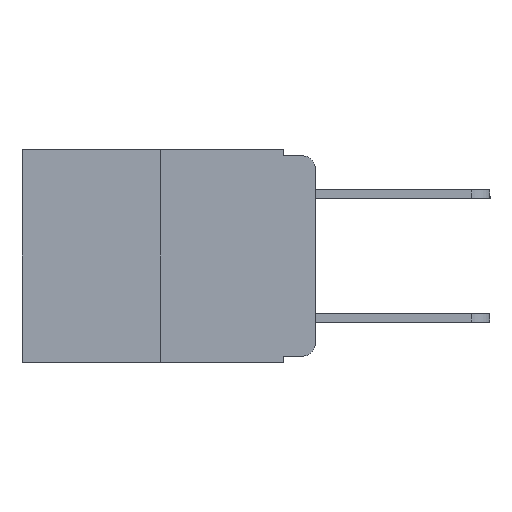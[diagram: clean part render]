
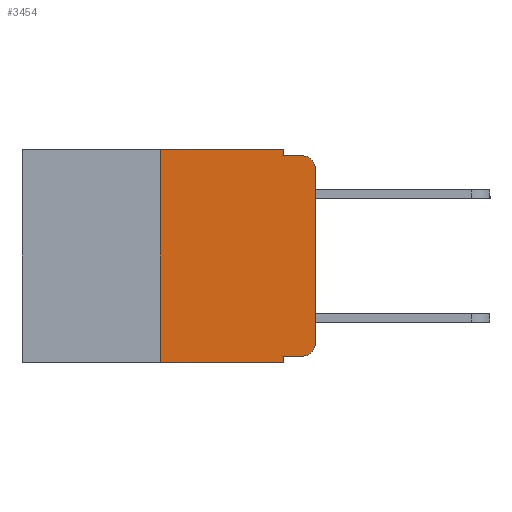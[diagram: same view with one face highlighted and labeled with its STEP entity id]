
A CAD part, left-side view. The second image highlights one B-rep face of the part: STEP entity #3454.
In plain terms, the highlighted planar face has unit normal (-1, 0, 0).
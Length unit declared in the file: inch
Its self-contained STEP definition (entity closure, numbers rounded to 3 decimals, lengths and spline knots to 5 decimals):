
#8 = CIRCLE ( 'NONE', #318, 0.02 ) ;
#318 = AXIS2_PLACEMENT_3D ( 'NONE', #6564, #405, #7449 ) ;
#341 = AXIS2_PLACEMENT_3D ( 'NONE', #9063, #3647, #9810 ) ;
#405 = DIRECTION ( 'NONE',  ( -1., 0., 0. ) ) ;
#509 = CARTESIAN_POINT ( 'NONE',  ( 0., 0.473, 0. ) ) ;
#791 = PLANE ( 'NONE',  #5399 ) ;
#895 = ORIENTED_EDGE ( 'NONE', *, *, #9069, .F. ) ;
#1317 = VERTEX_POINT ( 'NONE', #4248 ) ;
#1513 = VERTEX_POINT ( 'NONE', #5653 ) ;
#1748 = DIRECTION ( 'NONE',  ( 0., -1., 0. ) ) ;
#3040 = CARTESIAN_POINT ( 'NONE',  ( 0., 0.051, -0.343 ) ) ;
#3150 = LINE ( 'NONE', #4346, #7779 ) ;
#3346 = LINE ( 'NONE', #509, #10069 ) ;
#3454 = ADVANCED_FACE ( 'NONE', ( #8044 ), #791, .F. ) ;
#3488 = LINE ( 'NONE', #6900, #8137 ) ;
#3647 = DIRECTION ( 'NONE',  ( -1., 0., 0. ) ) ;
#3652 = LINE ( 'NONE', #7472, #8522 ) ;
#3686 = DIRECTION ( 'NONE',  ( 0., 0., -1. ) ) ;
#3776 = LINE ( 'NONE', #10562, #5989 ) ;
#3819 = EDGE_LOOP ( 'NONE', ( #5465, #4524, #5432, #895, #3895, #8691, #8847, #8886, #8919, #8930 ) ) ;
#3895 = ORIENTED_EDGE ( 'NONE', *, *, #9510, .F. ) ;
#4238 = VERTEX_POINT ( 'NONE', #5766 ) ;
#4248 = CARTESIAN_POINT ( 'NONE',  ( 0., 0.02, -0.01 ) ) ;
#4346 = CARTESIAN_POINT ( 'NONE',  ( 0., 0.473, -0.343 ) ) ;
#4377 = VERTEX_POINT ( 'NONE', #10115 ) ;
#4383 = VERTEX_POINT ( 'NONE', #6692 ) ;
#4524 = ORIENTED_EDGE ( 'NONE', *, *, #8584, .T. ) ;
#4530 = VERTEX_POINT ( 'NONE', #7323 ) ;
#4548 = LINE ( 'NONE', #5794, #7237 ) ;
#4826 = VECTOR ( 'NONE', #8921, 39.37008 ) ;
#5399 = AXIS2_PLACEMENT_3D ( 'NONE', #6695, #5581, #3686 ) ;
#5432 = ORIENTED_EDGE ( 'NONE', *, *, #8593, .F. ) ;
#5465 = ORIENTED_EDGE ( 'NONE', *, *, #9508, .T. ) ;
#5567 = LINE ( 'NONE', #10618, #7642 ) ;
#5581 = DIRECTION ( 'NONE',  ( 1., 0., 0. ) ) ;
#5653 = CARTESIAN_POINT ( 'NONE',  ( 0., 0.25, -0.343 ) ) ;
#5664 = DIRECTION ( 'NONE',  ( 0., 0., -1. ) ) ;
#5766 = CARTESIAN_POINT ( 'NONE',  ( 0., 0., -0.313 ) ) ;
#5794 = CARTESIAN_POINT ( 'NONE',  ( 0., 0.051, -0.333 ) ) ;
#5989 = VECTOR ( 'NONE', #11252, 39.37008 ) ;
#6550 = CIRCLE ( 'NONE', #341, 0.02 ) ;
#6564 = CARTESIAN_POINT ( 'NONE',  ( 0., 0.02, -0.313 ) ) ;
#6625 = DIRECTION ( 'NONE',  ( 0., 0., 1. ) ) ;
#6692 = CARTESIAN_POINT ( 'NONE',  ( 0., 0., -0.03 ) ) ;
#6695 = CARTESIAN_POINT ( 'NONE',  ( 0., 0.473, 0. ) ) ;
#6701 = CARTESIAN_POINT ( 'NONE',  ( 0., 0.25, 0. ) ) ;
#6900 = CARTESIAN_POINT ( 'NONE',  ( 0., 0.25, 0. ) ) ;
#7237 = VECTOR ( 'NONE', #11396, 39.37008 ) ;
#7323 = CARTESIAN_POINT ( 'NONE',  ( 0., 0.051, -0.333 ) ) ;
#7449 = DIRECTION ( 'NONE',  ( 0., 0., -1. ) ) ;
#7472 = CARTESIAN_POINT ( 'NONE',  ( 0., 0., 0. ) ) ;
#7642 = VECTOR ( 'NONE', #5664, 39.37008 ) ;
#7778 = DIRECTION ( 'NONE',  ( 0., 0., 1. ) ) ;
#7779 = VECTOR ( 'NONE', #11676, 39.37008 ) ;
#8044 = FACE_OUTER_BOUND ( 'NONE', #3819, .T. ) ;
#8137 = VECTOR ( 'NONE', #7778, 39.37008 ) ;
#8522 = VECTOR ( 'NONE', #6625, 39.37008 ) ;
#8584 = EDGE_CURVE ( 'NONE', #4383, #1317, #6550, .T. ) ;
#8593 = EDGE_CURVE ( 'NONE', #4377, #1317, #3776, .T. ) ;
#8608 = CARTESIAN_POINT ( 'NONE',  ( 0., 0.02, -0.333 ) ) ;
#8651 = EDGE_CURVE ( 'NONE', #11341, #4238, #8, .T. ) ;
#8657 = VERTEX_POINT ( 'NONE', #9890 ) ;
#8691 = ORIENTED_EDGE ( 'NONE', *, *, #9774, .F. ) ;
#8713 = EDGE_CURVE ( 'NONE', #4530, #11341, #4548, .T. ) ;
#8784 = VERTEX_POINT ( 'NONE', #3040 ) ;
#8847 = ORIENTED_EDGE ( 'NONE', *, *, #9018, .T. ) ;
#8886 = ORIENTED_EDGE ( 'NONE', *, *, #9384, .F. ) ;
#8919 = ORIENTED_EDGE ( 'NONE', *, *, #8713, .T. ) ;
#8921 = DIRECTION ( 'NONE',  ( 0., 0., -1. ) ) ;
#8930 = ORIENTED_EDGE ( 'NONE', *, *, #8651, .T. ) ;
#9018 = EDGE_CURVE ( 'NONE', #1513, #8784, #3150, .T. ) ;
#9063 = CARTESIAN_POINT ( 'NONE',  ( 0., 0.02, -0.03 ) ) ;
#9069 = EDGE_CURVE ( 'NONE', #8657, #4377, #11365, .T. ) ;
#9384 = EDGE_CURVE ( 'NONE', #4530, #8784, #5567, .T. ) ;
#9508 = EDGE_CURVE ( 'NONE', #4238, #4383, #3652, .T. ) ;
#9510 = EDGE_CURVE ( 'NONE', #9579, #8657, #3346, .T. ) ;
#9579 = VERTEX_POINT ( 'NONE', #6701 ) ;
#9774 = EDGE_CURVE ( 'NONE', #1513, #9579, #3488, .T. ) ;
#9810 = DIRECTION ( 'NONE',  ( 0., 0., -1. ) ) ;
#9890 = CARTESIAN_POINT ( 'NONE',  ( 0., 0.051, 0. ) ) ;
#10069 = VECTOR ( 'NONE', #1748, 39.37008 ) ;
#10115 = CARTESIAN_POINT ( 'NONE',  ( 0., 0.051, -0.01 ) ) ;
#10562 = CARTESIAN_POINT ( 'NONE',  ( 0., 0.051, -0.01 ) ) ;
#10618 = CARTESIAN_POINT ( 'NONE',  ( 0., 0.051, 0. ) ) ;
#11252 = DIRECTION ( 'NONE',  ( 0., -1., 0. ) ) ;
#11341 = VERTEX_POINT ( 'NONE', #8608 ) ;
#11365 = LINE ( 'NONE', #11738, #4826 ) ;
#11396 = DIRECTION ( 'NONE',  ( 0., -1., 0. ) ) ;
#11676 = DIRECTION ( 'NONE',  ( 0., -1., 0. ) ) ;
#11738 = CARTESIAN_POINT ( 'NONE',  ( 0., 0.051, 0. ) ) ;
